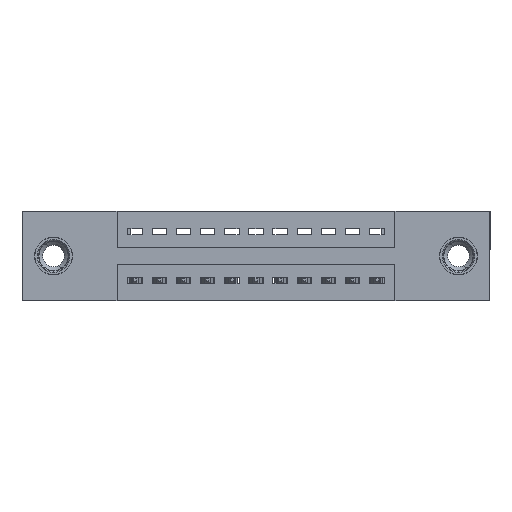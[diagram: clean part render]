
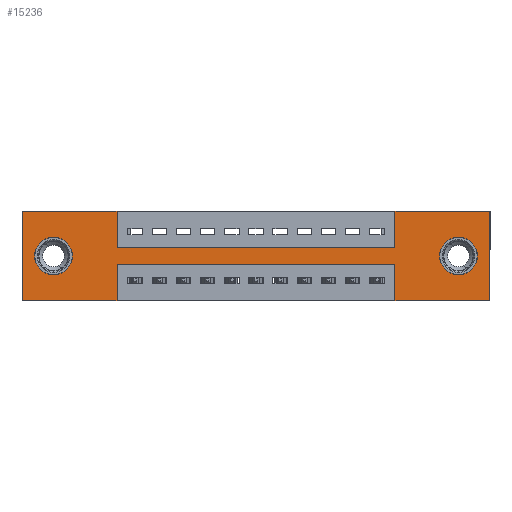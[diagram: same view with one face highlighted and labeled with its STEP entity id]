
A CAD part, front view. The second image highlights one B-rep face of the part: STEP entity #15236.
In plain terms, the highlighted planar face has unit normal (0, -1, 0).
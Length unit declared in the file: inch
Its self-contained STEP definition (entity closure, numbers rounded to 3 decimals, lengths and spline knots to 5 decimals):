
#214 = VERTEX_POINT ( 'NONE', #4495 ) ;
#316 = LINE ( 'NONE', #9428, #9879 ) ;
#475 = DIRECTION ( 'NONE',  ( 1., 0., 0. ) ) ;
#931 = LINE ( 'NONE', #2463, #15056 ) ;
#944 = VERTEX_POINT ( 'NONE', #12905 ) ;
#1009 = ORIENTED_EDGE ( 'NONE', *, *, #13205, .F. ) ;
#1106 = EDGE_CURVE ( 'NONE', #15248, #10833, #316, .T. ) ;
#1226 = LINE ( 'NONE', #12286, #16194 ) ;
#1358 = AXIS2_PLACEMENT_3D ( 'NONE', #12555, #16667, #10022 ) ;
#1412 = CARTESIAN_POINT ( 'NONE',  ( 0., 0., -0.37 ) ) ;
#1843 = VERTEX_POINT ( 'NONE', #10066 ) ;
#1866 = CIRCLE ( 'NONE', #2906, 0.078 ) ;
#1882 = CIRCLE ( 'NONE', #4471, 0.078 ) ;
#1929 = CARTESIAN_POINT ( 'NONE',  ( 0.3925, 0., -0.15 ) ) ;
#1958 = EDGE_CURVE ( 'NONE', #3059, #214, #931, .T. ) ;
#2126 = FACE_BOUND ( 'NONE', #8122, .T. ) ;
#2146 = EDGE_LOOP ( 'NONE', ( #11760, #4937 ) ) ;
#2463 = CARTESIAN_POINT ( 'NONE',  ( 0.3925, 0., -0.22 ) ) ;
#2624 = EDGE_CURVE ( 'NONE', #16876, #15366, #3825, .T. ) ;
#2741 = DIRECTION ( 'NONE',  ( 0., 0., -1. ) ) ;
#2863 = VECTOR ( 'NONE', #7831, 39.37008 ) ;
#2906 = AXIS2_PLACEMENT_3D ( 'NONE', #13427, #9219, #2741 ) ;
#3059 = VERTEX_POINT ( 'NONE', #5174 ) ;
#3271 = DIRECTION ( 'NONE',  ( 1., 0., 0. ) ) ;
#3391 = CARTESIAN_POINT ( 'NONE',  ( 0., 0., 0. ) ) ;
#3525 = CARTESIAN_POINT ( 'NONE',  ( 1.5425, 0., 0. ) ) ;
#3619 = VERTEX_POINT ( 'NONE', #7380 ) ;
#3797 = ORIENTED_EDGE ( 'NONE', *, *, #3980, .T. ) ;
#3799 = DIRECTION ( 'NONE',  ( -1., 0., 0. ) ) ;
#3825 = LINE ( 'NONE', #12337, #6710 ) ;
#3980 = EDGE_CURVE ( 'NONE', #5351, #1843, #16467, .T. ) ;
#4026 = CARTESIAN_POINT ( 'NONE',  ( 1.935, 0., 0. ) ) ;
#4332 = EDGE_LOOP ( 'NONE', ( #6484, #6805, #11127, #6147, #6191, #10397, #1009, #14652, #6391, #9119, #6301, #12601 ) ) ;
#4471 = AXIS2_PLACEMENT_3D ( 'NONE', #7154, #16423, #8416 ) ;
#4495 = CARTESIAN_POINT ( 'NONE',  ( 0.3925, 0., -0.22 ) ) ;
#4542 = LINE ( 'NONE', #4026, #10978 ) ;
#4652 = DIRECTION ( 'NONE',  ( -1., 0., 0. ) ) ;
#4806 = CARTESIAN_POINT ( 'NONE',  ( 0.3925, 0., 0. ) ) ;
#4937 = ORIENTED_EDGE ( 'NONE', *, *, #12061, .T. ) ;
#5092 = CARTESIAN_POINT ( 'NONE',  ( 0., 0., 0. ) ) ;
#5172 = VERTEX_POINT ( 'NONE', #12479 ) ;
#5174 = CARTESIAN_POINT ( 'NONE',  ( 1.5425, 0., -0.22 ) ) ;
#5351 = VERTEX_POINT ( 'NONE', #13575 ) ;
#5508 = CARTESIAN_POINT ( 'NONE',  ( 0., 0., -0.37 ) ) ;
#5695 = AXIS2_PLACEMENT_3D ( 'NONE', #5508, #8378, #13454 ) ;
#5737 = CARTESIAN_POINT ( 'NONE',  ( 1.5425, 0., -0.15 ) ) ;
#5969 = EDGE_CURVE ( 'NONE', #10833, #3059, #16815, .T. ) ;
#6074 = EDGE_CURVE ( 'NONE', #12044, #15248, #4542, .T. ) ;
#6147 = ORIENTED_EDGE ( 'NONE', *, *, #1106, .F. ) ;
#6166 = LINE ( 'NONE', #12665, #14290 ) ;
#6191 = ORIENTED_EDGE ( 'NONE', *, *, #6074, .F. ) ;
#6301 = ORIENTED_EDGE ( 'NONE', *, *, #11270, .F. ) ;
#6391 = ORIENTED_EDGE ( 'NONE', *, *, #2624, .F. ) ;
#6484 = ORIENTED_EDGE ( 'NONE', *, *, #16860, .F. ) ;
#6710 = VECTOR ( 'NONE', #10676, 39.37008 ) ;
#6805 = ORIENTED_EDGE ( 'NONE', *, *, #1958, .F. ) ;
#7154 = CARTESIAN_POINT ( 'NONE',  ( 0.13, 0., -0.185 ) ) ;
#7214 = CIRCLE ( 'NONE', #1358, 0.078 ) ;
#7380 = CARTESIAN_POINT ( 'NONE',  ( 0., 0., -0.37 ) ) ;
#7476 = CARTESIAN_POINT ( 'NONE',  ( 0.13, 0., -0.185 ) ) ;
#7617 = VERTEX_POINT ( 'NONE', #5092 ) ;
#7618 = CARTESIAN_POINT ( 'NONE',  ( 1.805, 0., -0.263 ) ) ;
#7831 = DIRECTION ( 'NONE',  ( 0., 0., 1. ) ) ;
#8122 = EDGE_LOOP ( 'NONE', ( #3797, #14459 ) ) ;
#8378 = DIRECTION ( 'NONE',  ( 0., -1., 0. ) ) ;
#8416 = DIRECTION ( 'NONE',  ( 0., 0., 1. ) ) ;
#8536 = FACE_OUTER_BOUND ( 'NONE', #4332, .T. ) ;
#9119 = ORIENTED_EDGE ( 'NONE', *, *, #16834, .F. ) ;
#9219 = DIRECTION ( 'NONE',  ( 0., 1., 0. ) ) ;
#9329 = LINE ( 'NONE', #15239, #15602 ) ;
#9428 = CARTESIAN_POINT ( 'NONE',  ( 0., 0., -0.37 ) ) ;
#9799 = FACE_BOUND ( 'NONE', #2146, .T. ) ;
#9844 = CARTESIAN_POINT ( 'NONE',  ( 1.935, 0., 0. ) ) ;
#9879 = VECTOR ( 'NONE', #4652, 39.37008 ) ;
#9935 = DIRECTION ( 'NONE',  ( 1., 0., 0. ) ) ;
#10022 = DIRECTION ( 'NONE',  ( 0., 0., -1. ) ) ;
#10066 = CARTESIAN_POINT ( 'NONE',  ( 0.13, 0., -0.263 ) ) ;
#10397 = ORIENTED_EDGE ( 'NONE', *, *, #11533, .F. ) ;
#10676 = DIRECTION ( 'NONE',  ( 0., 0., -1. ) ) ;
#10833 = VERTEX_POINT ( 'NONE', #16182 ) ;
#10978 = VECTOR ( 'NONE', #12137, 39.37008 ) ;
#11111 = CARTESIAN_POINT ( 'NONE',  ( 0., 0., 0. ) ) ;
#11127 = ORIENTED_EDGE ( 'NONE', *, *, #5969, .F. ) ;
#11144 = EDGE_CURVE ( 'NONE', #5172, #17123, #1866, .T. ) ;
#11187 = LINE ( 'NONE', #3391, #15346 ) ;
#11270 = EDGE_CURVE ( 'NONE', #3619, #7617, #1226, .T. ) ;
#11486 = DIRECTION ( 'NONE',  ( 0., 0., 1. ) ) ;
#11533 = EDGE_CURVE ( 'NONE', #13745, #12044, #11187, .T. ) ;
#11541 = DIRECTION ( 'NONE',  ( 0., 1., 0. ) ) ;
#11643 = LINE ( 'NONE', #11111, #12696 ) ;
#11760 = ORIENTED_EDGE ( 'NONE', *, *, #11144, .T. ) ;
#12044 = VERTEX_POINT ( 'NONE', #9844 ) ;
#12061 = EDGE_CURVE ( 'NONE', #17123, #5172, #7214, .T. ) ;
#12137 = DIRECTION ( 'NONE',  ( 0., 0., -1. ) ) ;
#12146 = PLANE ( 'NONE',  #5695 ) ;
#12286 = CARTESIAN_POINT ( 'NONE',  ( 0., 0., 0. ) ) ;
#12324 = CARTESIAN_POINT ( 'NONE',  ( 1.935, 0., -0.37 ) ) ;
#12337 = CARTESIAN_POINT ( 'NONE',  ( 0.3925, 0., 0. ) ) ;
#12472 = EDGE_CURVE ( 'NONE', #944, #3619, #16604, .T. ) ;
#12479 = CARTESIAN_POINT ( 'NONE',  ( 1.805, 0., -0.107 ) ) ;
#12555 = CARTESIAN_POINT ( 'NONE',  ( 1.805, 0., -0.185 ) ) ;
#12601 = ORIENTED_EDGE ( 'NONE', *, *, #12472, .F. ) ;
#12665 = CARTESIAN_POINT ( 'NONE',  ( 1.5425, 0., 0. ) ) ;
#12696 = VECTOR ( 'NONE', #9935, 39.37008 ) ;
#12905 = CARTESIAN_POINT ( 'NONE',  ( 0.3925, 0., -0.37 ) ) ;
#13190 = VERTEX_POINT ( 'NONE', #5737 ) ;
#13205 = EDGE_CURVE ( 'NONE', #13190, #13745, #6166, .T. ) ;
#13329 = LINE ( 'NONE', #1929, #16453 ) ;
#13419 = AXIS2_PLACEMENT_3D ( 'NONE', #7476, #11541, #11486 ) ;
#13427 = CARTESIAN_POINT ( 'NONE',  ( 1.805, 0., -0.185 ) ) ;
#13454 = DIRECTION ( 'NONE',  ( 0., 0., -1. ) ) ;
#13575 = CARTESIAN_POINT ( 'NONE',  ( 0.13, 0., -0.107 ) ) ;
#13745 = VERTEX_POINT ( 'NONE', #3525 ) ;
#14290 = VECTOR ( 'NONE', #15259, 39.37008 ) ;
#14459 = ORIENTED_EDGE ( 'NONE', *, *, #16807, .T. ) ;
#14600 = DIRECTION ( 'NONE',  ( -1., 0., 0. ) ) ;
#14652 = ORIENTED_EDGE ( 'NONE', *, *, #16096, .F. ) ;
#14714 = VECTOR ( 'NONE', #14600, 39.37008 ) ;
#15056 = VECTOR ( 'NONE', #3799, 39.37008 ) ;
#15236 = ADVANCED_FACE ( 'NONE', ( #9799, #2126, #8536 ), #12146, .T. ) ;
#15239 = CARTESIAN_POINT ( 'NONE',  ( 0.3925, 0., -0.37 ) ) ;
#15248 = VERTEX_POINT ( 'NONE', #12324 ) ;
#15259 = DIRECTION ( 'NONE',  ( 0., 0., 1. ) ) ;
#15346 = VECTOR ( 'NONE', #475, 39.37008 ) ;
#15366 = VERTEX_POINT ( 'NONE', #16491 ) ;
#15602 = VECTOR ( 'NONE', #16701, 39.37008 ) ;
#15987 = CARTESIAN_POINT ( 'NONE',  ( 1.5425, 0., -0.37 ) ) ;
#16096 = EDGE_CURVE ( 'NONE', #15366, #13190, #13329, .T. ) ;
#16182 = CARTESIAN_POINT ( 'NONE',  ( 1.5425, 0., -0.37 ) ) ;
#16194 = VECTOR ( 'NONE', #16225, 39.37008 ) ;
#16225 = DIRECTION ( 'NONE',  ( 0., 0., 1. ) ) ;
#16423 = DIRECTION ( 'NONE',  ( 0., 1., 0. ) ) ;
#16453 = VECTOR ( 'NONE', #3271, 39.37008 ) ;
#16467 = CIRCLE ( 'NONE', #13419, 0.078 ) ;
#16491 = CARTESIAN_POINT ( 'NONE',  ( 0.3925, 0., -0.15 ) ) ;
#16604 = LINE ( 'NONE', #1412, #14714 ) ;
#16667 = DIRECTION ( 'NONE',  ( 0., 1., 0. ) ) ;
#16701 = DIRECTION ( 'NONE',  ( 0., 0., -1. ) ) ;
#16807 = EDGE_CURVE ( 'NONE', #1843, #5351, #1882, .T. ) ;
#16815 = LINE ( 'NONE', #15987, #2863 ) ;
#16834 = EDGE_CURVE ( 'NONE', #7617, #16876, #11643, .T. ) ;
#16860 = EDGE_CURVE ( 'NONE', #214, #944, #9329, .T. ) ;
#16876 = VERTEX_POINT ( 'NONE', #4806 ) ;
#17123 = VERTEX_POINT ( 'NONE', #7618 ) ;
